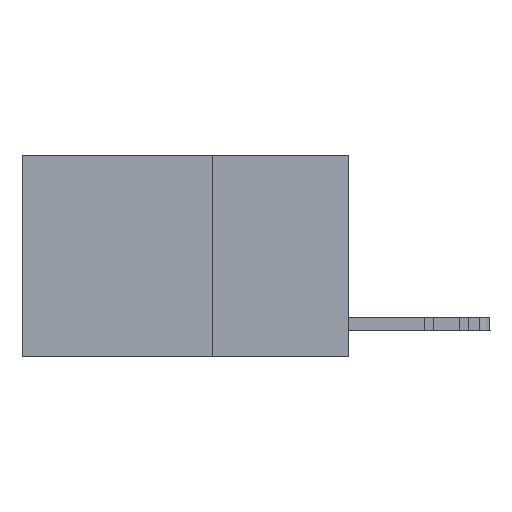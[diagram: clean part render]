
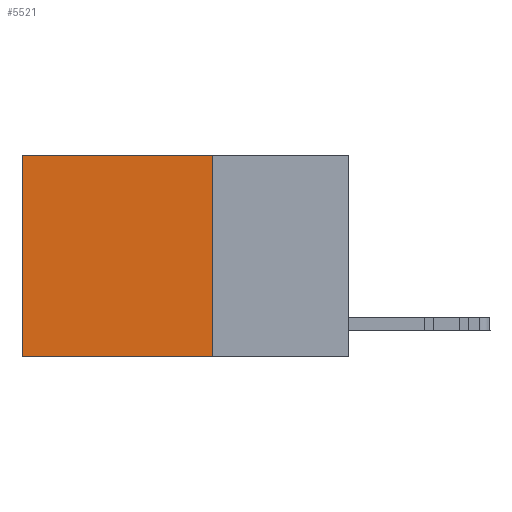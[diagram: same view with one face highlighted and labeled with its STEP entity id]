
A CAD part, left-side view. The second image highlights one B-rep face of the part: STEP entity #5521.
In plain terms, the highlighted planar face has unit normal (-1, 0, 0).
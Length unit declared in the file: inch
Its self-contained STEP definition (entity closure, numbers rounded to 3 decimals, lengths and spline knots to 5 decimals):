
#475 = LINE ( 'NONE', #4796, #25190 ) ;
#673 = DIRECTION ( 'NONE',  ( 0., 1., 0. ) ) ;
#1598 = LINE ( 'NONE', #6055, #16255 ) ;
#2461 = VERTEX_POINT ( 'NONE', #16795 ) ;
#2694 = DIRECTION ( 'NONE',  ( 0., 0., -1. ) ) ;
#2722 = CARTESIAN_POINT ( 'NONE',  ( 0.2625, 0.25, 0. ) ) ;
#2947 = AXIS2_PLACEMENT_3D ( 'NONE', #17716, #6821, #13454 ) ;
#4213 = VECTOR ( 'NONE', #11188, 39.37008 ) ;
#4796 = CARTESIAN_POINT ( 'NONE',  ( 0.2625, 0.6, 0. ) ) ;
#5521 = ADVANCED_FACE ( 'NONE', ( #17581 ), #17852, .F. ) ;
#6055 = CARTESIAN_POINT ( 'NONE',  ( 0.2625, 0.25, -0.37 ) ) ;
#6320 = DIRECTION ( 'NONE',  ( 0., 1., 0. ) ) ;
#6821 = DIRECTION ( 'NONE',  ( 1., 0., 0. ) ) ;
#6938 = CARTESIAN_POINT ( 'NONE',  ( 0.2625, 0.25, 0. ) ) ;
#6942 = ORIENTED_EDGE ( 'NONE', *, *, #15326, .F. ) ;
#7716 = VERTEX_POINT ( 'NONE', #6938 ) ;
#8119 = EDGE_CURVE ( 'NONE', #15038, #20809, #475, .T. ) ;
#8993 = VECTOR ( 'NONE', #673, 39.37008 ) ;
#9996 = ORIENTED_EDGE ( 'NONE', *, *, #13333, .T. ) ;
#11188 = DIRECTION ( 'NONE',  ( 0., 0., -1. ) ) ;
#13333 = EDGE_CURVE ( 'NONE', #7716, #15038, #15608, .T. ) ;
#13454 = DIRECTION ( 'NONE',  ( 0., 0., -1. ) ) ;
#15038 = VERTEX_POINT ( 'NONE', #15443 ) ;
#15326 = EDGE_CURVE ( 'NONE', #2461, #20809, #1598, .T. ) ;
#15443 = CARTESIAN_POINT ( 'NONE',  ( 0.2625, 0.6, 0. ) ) ;
#15608 = LINE ( 'NONE', #22510, #8993 ) ;
#16255 = VECTOR ( 'NONE', #6320, 39.37008 ) ;
#16795 = CARTESIAN_POINT ( 'NONE',  ( 0.2625, 0.25, -0.37 ) ) ;
#17581 = FACE_OUTER_BOUND ( 'NONE', #21855, .T. ) ;
#17716 = CARTESIAN_POINT ( 'NONE',  ( 0.2625, 0.25, 0. ) ) ;
#17852 = PLANE ( 'NONE',  #2947 ) ;
#19333 = EDGE_CURVE ( 'NONE', #7716, #2461, #22063, .T. ) ;
#20073 = ORIENTED_EDGE ( 'NONE', *, *, #8119, .T. ) ;
#20111 = CARTESIAN_POINT ( 'NONE',  ( 0.2625, 0.6, -0.37 ) ) ;
#20809 = VERTEX_POINT ( 'NONE', #20111 ) ;
#21855 = EDGE_LOOP ( 'NONE', ( #20073, #6942, #22431, #9996 ) ) ;
#22063 = LINE ( 'NONE', #2722, #4213 ) ;
#22431 = ORIENTED_EDGE ( 'NONE', *, *, #19333, .F. ) ;
#22510 = CARTESIAN_POINT ( 'NONE',  ( 0.2625, 0.25, 0. ) ) ;
#25190 = VECTOR ( 'NONE', #2694, 39.37008 ) ;
